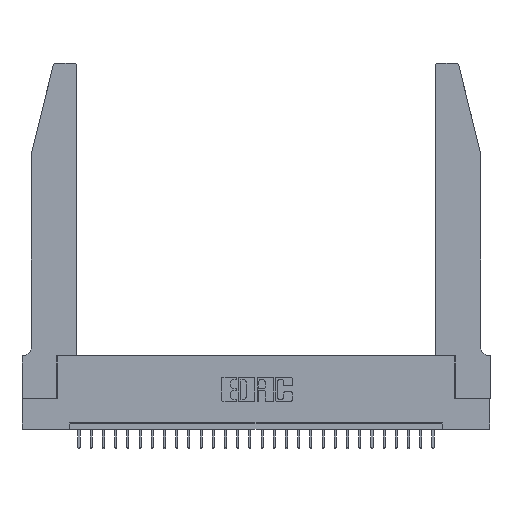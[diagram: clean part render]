
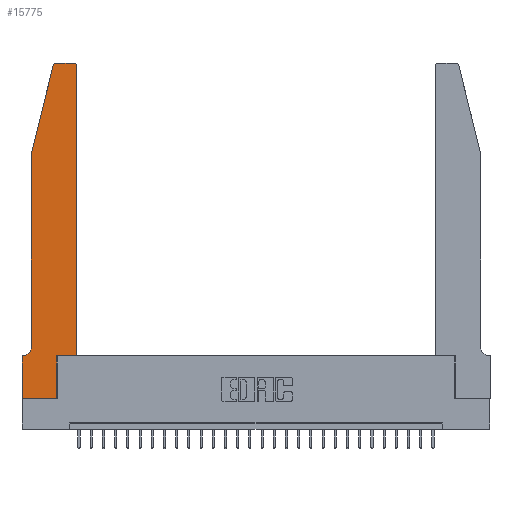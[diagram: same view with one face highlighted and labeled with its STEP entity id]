
A CAD part, top view. The second image highlights one B-rep face of the part: STEP entity #15775.
In plain terms, the highlighted planar face has unit normal (0, 0, 1).
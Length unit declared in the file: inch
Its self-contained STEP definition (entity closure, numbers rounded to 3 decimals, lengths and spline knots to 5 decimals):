
#388 = AXIS2_PLACEMENT_3D ( 'NONE', #28271, #23855, #17460 ) ;
#401 = EDGE_CURVE ( 'NONE', #10527, #4007, #25624, .T. ) ;
#494 = CARTESIAN_POINT ( 'NONE',  ( 0.2865, 0., 0.37 ) ) ;
#592 = CARTESIAN_POINT ( 'NONE',  ( 0.4505, 2.72, 0.37 ) ) ;
#640 = EDGE_CURVE ( 'NONE', #27322, #3493, #28050, .T. ) ;
#812 = CARTESIAN_POINT ( 'NONE',  ( 0.4505, 0.35, 0.37 ) ) ;
#1185 = CARTESIAN_POINT ( 'NONE',  ( 0.4505, 0.35, 0.37 ) ) ;
#1463 = DIRECTION ( 'NONE',  ( 1., 0., 0. ) ) ;
#1568 = DIRECTION ( 'NONE',  ( 1., 0., 0. ) ) ;
#2234 = DIRECTION ( 'NONE',  ( 0., 0., 1. ) ) ;
#2237 = VERTEX_POINT ( 'NONE', #7067 ) ;
#2246 = VERTEX_POINT ( 'NONE', #25910 ) ;
#2566 = VERTEX_POINT ( 'NONE', #26806 ) ;
#2587 = ORIENTED_EDGE ( 'NONE', *, *, #9863, .T. ) ;
#2727 = LINE ( 'NONE', #20184, #10136 ) ;
#3470 = EDGE_CURVE ( 'NONE', #2566, #27322, #23378, .T. ) ;
#3493 = VERTEX_POINT ( 'NONE', #8712 ) ;
#3999 = CIRCLE ( 'NONE', #9042, 0.07 ) ;
#4007 = VERTEX_POINT ( 'NONE', #592 ) ;
#4585 = EDGE_CURVE ( 'NONE', #4007, #5436, #26840, .T. ) ;
#4672 = EDGE_CURVE ( 'NONE', #27811, #28675, #20128, .T. ) ;
#5012 = ORIENTED_EDGE ( 'NONE', *, *, #25265, .T. ) ;
#5436 = VERTEX_POINT ( 'NONE', #24432 ) ;
#5543 = LINE ( 'NONE', #14122, #19220 ) ;
#5578 = CARTESIAN_POINT ( 'NONE',  ( 0.284, 2.75, 0.37 ) ) ;
#6268 = ORIENTED_EDGE ( 'NONE', *, *, #4585, .T. ) ;
#6284 = CARTESIAN_POINT ( 'NONE',  ( 0.0755, 2., 0.37 ) ) ;
#6310 = VERTEX_POINT ( 'NONE', #12985 ) ;
#7067 = CARTESIAN_POINT ( 'NONE',  ( 0.25487, 2.72718, 0.37 ) ) ;
#7501 = DIRECTION ( 'NONE',  ( -1., 0., 0. ) ) ;
#8047 = DIRECTION ( 'NONE',  ( 1., 0., 0. ) ) ;
#8052 = CARTESIAN_POINT ( 'NONE',  ( 0.4505, 0.35, 0.37 ) ) ;
#8238 = VECTOR ( 'NONE', #28194, 39.37008 ) ;
#8331 = VECTOR ( 'NONE', #8047, 39.37008 ) ;
#8689 = DIRECTION ( 'NONE',  ( 0., 1., 0. ) ) ;
#8712 = CARTESIAN_POINT ( 'NONE',  ( 0.2865, 0.35, 0.37 ) ) ;
#9042 = AXIS2_PLACEMENT_3D ( 'NONE', #26274, #28052, #21371 ) ;
#9142 = CARTESIAN_POINT ( 'NONE',  ( 0.0755, 0.42, 0.37 ) ) ;
#9498 = VECTOR ( 'NONE', #9755, 39.37008 ) ;
#9630 = LINE ( 'NONE', #25049, #27502 ) ;
#9753 = ORIENTED_EDGE ( 'NONE', *, *, #3470, .T. ) ;
#9755 = DIRECTION ( 'NONE',  ( 0., 1., 0. ) ) ;
#9863 = EDGE_CURVE ( 'NONE', #5436, #16781, #9630, .T. ) ;
#10136 = VECTOR ( 'NONE', #17924, 39.37008 ) ;
#10527 = VERTEX_POINT ( 'NONE', #8052 ) ;
#11630 = ORIENTED_EDGE ( 'NONE', *, *, #27643, .T. ) ;
#11801 = ORIENTED_EDGE ( 'NONE', *, *, #17018, .T. ) ;
#12579 = PLANE ( 'NONE',  #16678 ) ;
#12848 = FACE_OUTER_BOUND ( 'NONE', #17328, .T. ) ;
#12985 = CARTESIAN_POINT ( 'NONE',  ( 0., 0.35, 0.37 ) ) ;
#13198 = EDGE_CURVE ( 'NONE', #2246, #6310, #26593, .T. ) ;
#14122 = CARTESIAN_POINT ( 'NONE',  ( 0.0755, 2., 0.37 ) ) ;
#14191 = ORIENTED_EDGE ( 'NONE', *, *, #401, .T. ) ;
#14314 = CIRCLE ( 'NONE', #388, 0.03 ) ;
#14952 = ORIENTED_EDGE ( 'NONE', *, *, #16794, .T. ) ;
#15381 = DIRECTION ( 'NONE',  ( -1., 0., 0. ) ) ;
#15718 = VECTOR ( 'NONE', #15381, 39.37008 ) ;
#15775 = ADVANCED_FACE ( 'NONE', ( #12848 ), #12579, .T. ) ;
#15822 = ORIENTED_EDGE ( 'NONE', *, *, #640, .T. ) ;
#16147 = DIRECTION ( 'NONE',  ( -0.239, -0.971, 0. ) ) ;
#16678 = AXIS2_PLACEMENT_3D ( 'NONE', #19582, #19275, #1568 ) ;
#16781 = VERTEX_POINT ( 'NONE', #5578 ) ;
#16794 = EDGE_CURVE ( 'NONE', #3493, #10527, #26950, .T. ) ;
#17018 = EDGE_CURVE ( 'NONE', #16781, #2237, #14314, .T. ) ;
#17328 = EDGE_LOOP ( 'NONE', ( #2587, #11801, #5012, #17368, #11630, #21501, #17562, #9753, #15822, #14952, #14191, #6268 ) ) ;
#17368 = ORIENTED_EDGE ( 'NONE', *, *, #4672, .T. ) ;
#17460 = DIRECTION ( 'NONE',  ( 1., 0., 0. ) ) ;
#17562 = ORIENTED_EDGE ( 'NONE', *, *, #25499, .T. ) ;
#17924 = DIRECTION ( 'NONE',  ( 0., -1., 0. ) ) ;
#19220 = VECTOR ( 'NONE', #16147, 39.37008 ) ;
#19275 = DIRECTION ( 'NONE',  ( 0., 0., 1. ) ) ;
#19582 = CARTESIAN_POINT ( 'NONE',  ( 0., 0.35, 0.37 ) ) ;
#20128 = LINE ( 'NONE', #21723, #8238 ) ;
#20184 = CARTESIAN_POINT ( 'NONE',  ( 0., 0., 0.37 ) ) ;
#20645 = VECTOR ( 'NONE', #8689, 39.37008 ) ;
#20993 = VECTOR ( 'NONE', #25481, 39.37008 ) ;
#21371 = DIRECTION ( 'NONE',  ( -1., 0., 0. ) ) ;
#21501 = ORIENTED_EDGE ( 'NONE', *, *, #13198, .T. ) ;
#21723 = CARTESIAN_POINT ( 'NONE',  ( 0.0755, 2., 0.37 ) ) ;
#23378 = LINE ( 'NONE', #26713, #8331 ) ;
#23855 = DIRECTION ( 'NONE',  ( 0., 0., 1. ) ) ;
#24103 = CARTESIAN_POINT ( 'NONE',  ( 0.0755, 0.35, 0.37 ) ) ;
#24432 = CARTESIAN_POINT ( 'NONE',  ( 0.4205, 2.75, 0.37 ) ) ;
#25049 = CARTESIAN_POINT ( 'NONE',  ( 0.2605, 2.75, 0.37 ) ) ;
#25265 = EDGE_CURVE ( 'NONE', #2237, #27811, #5543, .T. ) ;
#25481 = DIRECTION ( 'NONE',  ( 1., 0., 0. ) ) ;
#25499 = EDGE_CURVE ( 'NONE', #6310, #2566, #2727, .T. ) ;
#25624 = LINE ( 'NONE', #812, #9498 ) ;
#25910 = CARTESIAN_POINT ( 'NONE',  ( 0.0055, 0.35, 0.37 ) ) ;
#26274 = CARTESIAN_POINT ( 'NONE',  ( 0.0055, 0.42, 0.37 ) ) ;
#26356 = CARTESIAN_POINT ( 'NONE',  ( 0.4205, 2.72, 0.37 ) ) ;
#26593 = LINE ( 'NONE', #24103, #15718 ) ;
#26713 = CARTESIAN_POINT ( 'NONE',  ( 0., 0., 0.37 ) ) ;
#26806 = CARTESIAN_POINT ( 'NONE',  ( 0., 0., 0.37 ) ) ;
#26840 = CIRCLE ( 'NONE', #28590, 0.03 ) ;
#26950 = LINE ( 'NONE', #1185, #20993 ) ;
#27322 = VERTEX_POINT ( 'NONE', #494 ) ;
#27502 = VECTOR ( 'NONE', #7501, 39.37008 ) ;
#27643 = EDGE_CURVE ( 'NONE', #28675, #2246, #3999, .T. ) ;
#27811 = VERTEX_POINT ( 'NONE', #6284 ) ;
#28050 = LINE ( 'NONE', #28663, #20645 ) ;
#28052 = DIRECTION ( 'NONE',  ( 0., 0., -1. ) ) ;
#28194 = DIRECTION ( 'NONE',  ( 0., -1., 0. ) ) ;
#28271 = CARTESIAN_POINT ( 'NONE',  ( 0.284, 2.72, 0.37 ) ) ;
#28590 = AXIS2_PLACEMENT_3D ( 'NONE', #26356, #2234, #1463 ) ;
#28663 = CARTESIAN_POINT ( 'NONE',  ( 0.2865, 0.35, 0.37 ) ) ;
#28675 = VERTEX_POINT ( 'NONE', #9142 ) ;
